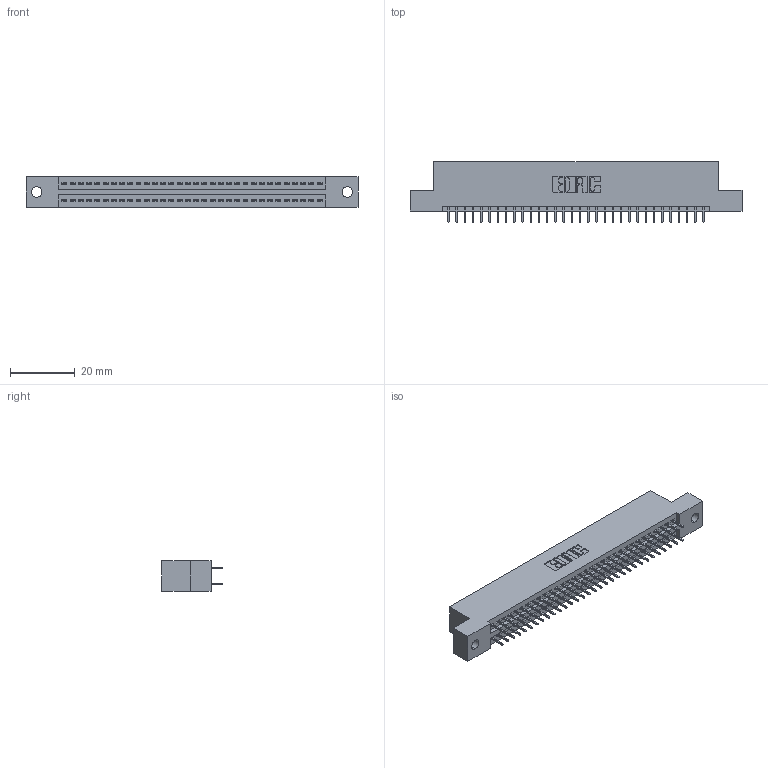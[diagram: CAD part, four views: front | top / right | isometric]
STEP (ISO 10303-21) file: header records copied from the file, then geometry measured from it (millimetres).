
FILE_DESCRIPTION (( 'STEP AP203' ), '1' );
FILE_NAME ('895-064-525-202.STEP', '2020-09-28T10:22:47', ( '' ), ( '' ), 'SwSTEP 2.0', 'SolidWorks 2020', '' );
FILE_SCHEMA (( 'CONFIG_CONTROL_DESIGN' ));
Length unit declared in the file: inch
Products named in the file (3): 345-292-001_345-293-125; 895-064-525-202; 845 Part_Flush Mounting Lugs - 0.128 Dia
Assembly tree (65 placements, depth 2):
  895-064-525-202
    845 Part_Flush Mounting Lugs - 0.128 Dia
    345-292-001_345-293-125  x64
Bounding box: 102.49 x 18.72 x 9.4 mm (x, y, z)
Volume: 9721 mm3; surface area: 13585.5 mm2
Topology: 65 solids, 65 shells, 3582 faces, 10133 edges, 6498 vertices
Faces by surface type: plane 2576, cylinder 1006
Entity records: 26531 total; most frequent: CARTESIAN_POINT 4456, ORIENTED_EDGE 4390, DIRECTION 3943, EDGE_CURVE 2195, LINE 1939, VECTOR 1939, VERTEX_POINT 1458, AXIS2_PLACEMENT_3D 1002
